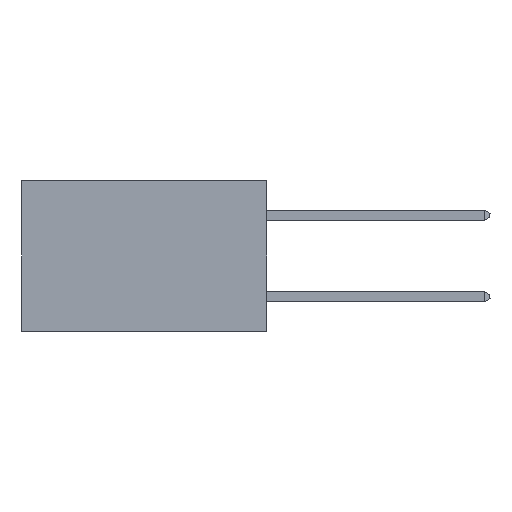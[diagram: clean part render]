
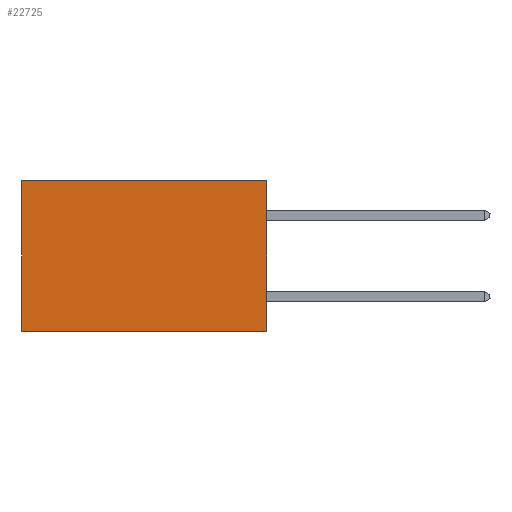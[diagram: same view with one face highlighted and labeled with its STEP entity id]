
A CAD part, left-side view. The second image highlights one B-rep face of the part: STEP entity #22725.
In plain terms, the highlighted planar face has unit normal (-1, 0, 0).
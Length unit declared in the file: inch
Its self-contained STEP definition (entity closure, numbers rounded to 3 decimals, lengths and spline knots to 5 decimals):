
#1172 = VERTEX_POINT ( 'NONE', #8597 ) ;
#1580 = CARTESIAN_POINT ( 'NONE',  ( 0.2875, 0., 0. ) ) ;
#5643 = CARTESIAN_POINT ( 'NONE',  ( 0.2875, 0., 0. ) ) ;
#6239 = VECTOR ( 'NONE', #17219, 39.37008 ) ;
#6276 = LINE ( 'NONE', #32289, #30150 ) ;
#6404 = PLANE ( 'NONE',  #28768 ) ;
#8597 = CARTESIAN_POINT ( 'NONE',  ( 0.2875, 0.6, -0.37 ) ) ;
#11748 = DIRECTION ( 'NONE',  ( 0., 1., 0. ) ) ;
#11996 = EDGE_CURVE ( 'NONE', #23475, #1172, #31717, .T. ) ;
#14523 = DIRECTION ( 'NONE',  ( 0., 0., -1. ) ) ;
#15449 = ORIENTED_EDGE ( 'NONE', *, *, #22427, .F. ) ;
#15691 = DIRECTION ( 'NONE',  ( 0., 0., -1. ) ) ;
#15887 = CARTESIAN_POINT ( 'NONE',  ( 0.2875, 0., -0.37 ) ) ;
#16821 = VERTEX_POINT ( 'NONE', #23636 ) ;
#17219 = DIRECTION ( 'NONE',  ( 0., 0., -1. ) ) ;
#17452 = EDGE_CURVE ( 'NONE', #16821, #1172, #23240, .T. ) ;
#18131 = ORIENTED_EDGE ( 'NONE', *, *, #11996, .F. ) ;
#19634 = ORIENTED_EDGE ( 'NONE', *, *, #17452, .T. ) ;
#22427 = EDGE_CURVE ( 'NONE', #27266, #23475, #6276, .T. ) ;
#22725 = ADVANCED_FACE ( 'NONE', ( #34745 ), #6404, .F. ) ;
#23240 = LINE ( 'NONE', #26148, #6239 ) ;
#23475 = VERTEX_POINT ( 'NONE', #15887 ) ;
#23636 = CARTESIAN_POINT ( 'NONE',  ( 0.2875, 0.6, 0. ) ) ;
#23907 = VECTOR ( 'NONE', #29051, 39.37008 ) ;
#24566 = CARTESIAN_POINT ( 'NONE',  ( 0.2875, 0., 0. ) ) ;
#24861 = LINE ( 'NONE', #5643, #31739 ) ;
#26148 = CARTESIAN_POINT ( 'NONE',  ( 0.2875, 0.6, 0. ) ) ;
#26834 = EDGE_CURVE ( 'NONE', #27266, #16821, #24861, .T. ) ;
#27266 = VERTEX_POINT ( 'NONE', #1580 ) ;
#28768 = AXIS2_PLACEMENT_3D ( 'NONE', #24566, #33436, #15691 ) ;
#29051 = DIRECTION ( 'NONE',  ( 0., 1., 0. ) ) ;
#30127 = EDGE_LOOP ( 'NONE', ( #19634, #18131, #15449, #33613 ) ) ;
#30150 = VECTOR ( 'NONE', #14523, 39.37008 ) ;
#31717 = LINE ( 'NONE', #34823, #23907 ) ;
#31739 = VECTOR ( 'NONE', #11748, 39.37008 ) ;
#32289 = CARTESIAN_POINT ( 'NONE',  ( 0.2875, 0., 0. ) ) ;
#33436 = DIRECTION ( 'NONE',  ( 1., 0., 0. ) ) ;
#33613 = ORIENTED_EDGE ( 'NONE', *, *, #26834, .T. ) ;
#34745 = FACE_OUTER_BOUND ( 'NONE', #30127, .T. ) ;
#34823 = CARTESIAN_POINT ( 'NONE',  ( 0.2875, 0., -0.37 ) ) ;
